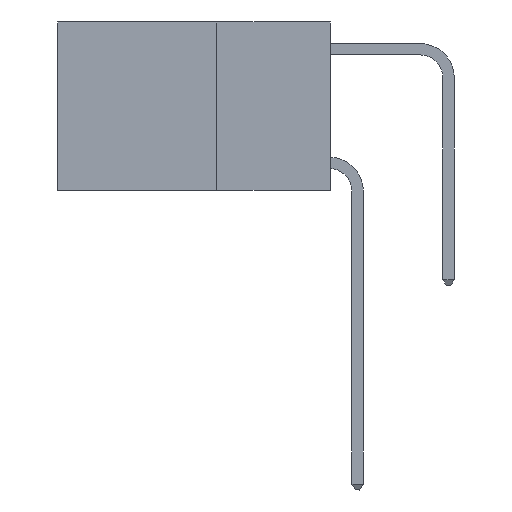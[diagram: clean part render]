
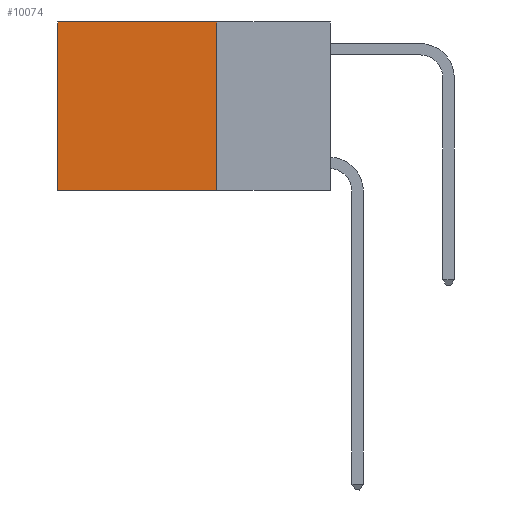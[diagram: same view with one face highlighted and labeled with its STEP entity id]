
A CAD part, left-side view. The second image highlights one B-rep face of the part: STEP entity #10074.
In plain terms, the highlighted planar face has unit normal (-1, 0, 0).
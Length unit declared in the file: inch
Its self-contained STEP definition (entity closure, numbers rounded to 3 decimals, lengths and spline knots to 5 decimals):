
#46 = CARTESIAN_POINT ( 'NONE',  ( 0.2625, 0.25, 0. ) ) ;
#238 = EDGE_CURVE ( 'NONE', #1097, #23597, #12131, .T. ) ;
#880 = CARTESIAN_POINT ( 'NONE',  ( 0.2625, 0.25, -0.37 ) ) ;
#1097 = VERTEX_POINT ( 'NONE', #880 ) ;
#2764 = LINE ( 'NONE', #9998, #7425 ) ;
#3077 = LINE ( 'NONE', #20955, #23642 ) ;
#4104 = PLANE ( 'NONE',  #13595 ) ;
#4213 = VERTEX_POINT ( 'NONE', #46 ) ;
#4793 = ORIENTED_EDGE ( 'NONE', *, *, #238, .F. ) ;
#5159 = VECTOR ( 'NONE', #15262, 39.37008 ) ;
#5821 = VERTEX_POINT ( 'NONE', #12479 ) ;
#7425 = VECTOR ( 'NONE', #11932, 39.37008 ) ;
#7483 = DIRECTION ( 'NONE',  ( 0., 1., 0. ) ) ;
#8049 = DIRECTION ( 'NONE',  ( 1., 0., 0. ) ) ;
#8506 = VECTOR ( 'NONE', #14338, 39.37008 ) ;
#9880 = EDGE_CURVE ( 'NONE', #4213, #5821, #3077, .T. ) ;
#9998 = CARTESIAN_POINT ( 'NONE',  ( 0.2625, 0.25, 0. ) ) ;
#10074 = ADVANCED_FACE ( 'NONE', ( #14689 ), #4104, .F. ) ;
#10567 = CARTESIAN_POINT ( 'NONE',  ( 0.2625, 0.6, 0. ) ) ;
#11932 = DIRECTION ( 'NONE',  ( 0., 0., -1. ) ) ;
#12131 = LINE ( 'NONE', #20972, #5159 ) ;
#12479 = CARTESIAN_POINT ( 'NONE',  ( 0.2625, 0.6, 0. ) ) ;
#12842 = EDGE_CURVE ( 'NONE', #5821, #23597, #14218, .T. ) ;
#13595 = AXIS2_PLACEMENT_3D ( 'NONE', #15727, #8049, #21520 ) ;
#14010 = EDGE_LOOP ( 'NONE', ( #21065, #4793, #17816, #20219 ) ) ;
#14218 = LINE ( 'NONE', #10567, #8506 ) ;
#14338 = DIRECTION ( 'NONE',  ( 0., 0., -1. ) ) ;
#14689 = FACE_OUTER_BOUND ( 'NONE', #14010, .T. ) ;
#15262 = DIRECTION ( 'NONE',  ( 0., 1., 0. ) ) ;
#15727 = CARTESIAN_POINT ( 'NONE',  ( 0.2625, 0.25, 0. ) ) ;
#16655 = EDGE_CURVE ( 'NONE', #4213, #1097, #2764, .T. ) ;
#16873 = CARTESIAN_POINT ( 'NONE',  ( 0.2625, 0.6, -0.37 ) ) ;
#17816 = ORIENTED_EDGE ( 'NONE', *, *, #16655, .F. ) ;
#20219 = ORIENTED_EDGE ( 'NONE', *, *, #9880, .T. ) ;
#20955 = CARTESIAN_POINT ( 'NONE',  ( 0.2625, 0.25, 0. ) ) ;
#20972 = CARTESIAN_POINT ( 'NONE',  ( 0.2625, 0.25, -0.37 ) ) ;
#21065 = ORIENTED_EDGE ( 'NONE', *, *, #12842, .T. ) ;
#21520 = DIRECTION ( 'NONE',  ( 0., 0., -1. ) ) ;
#23597 = VERTEX_POINT ( 'NONE', #16873 ) ;
#23642 = VECTOR ( 'NONE', #7483, 39.37008 ) ;
